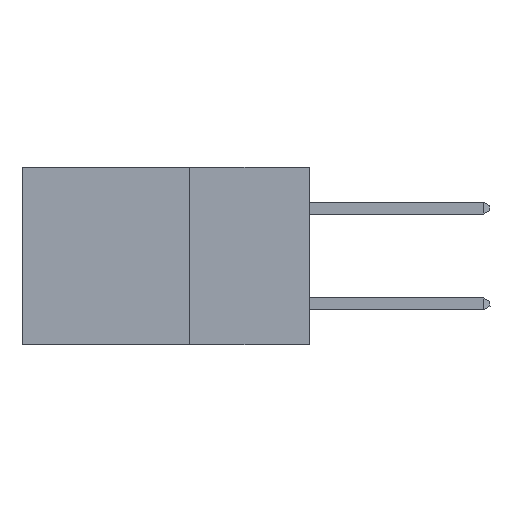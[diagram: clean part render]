
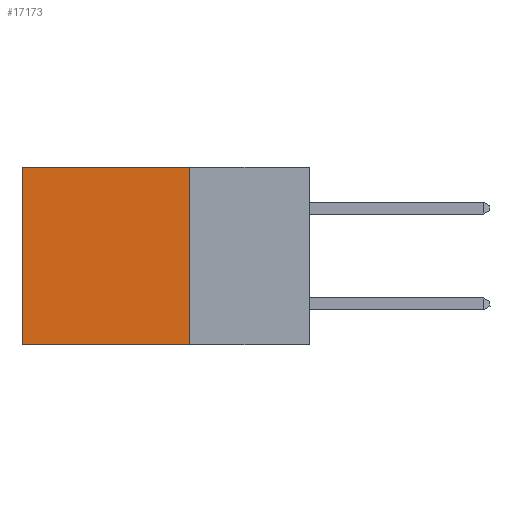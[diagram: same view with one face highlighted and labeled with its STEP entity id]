
A CAD part, left-side view. The second image highlights one B-rep face of the part: STEP entity #17173.
In plain terms, the highlighted planar face has unit normal (-1, 0, 0).
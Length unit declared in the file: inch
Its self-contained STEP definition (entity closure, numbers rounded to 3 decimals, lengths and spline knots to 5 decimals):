
#401 = CARTESIAN_POINT ( 'NONE',  ( 0.2875, 0.25, -0.37 ) ) ;
#508 = EDGE_CURVE ( 'NONE', #2702, #4521, #17261, .T. ) ;
#776 = VERTEX_POINT ( 'NONE', #10288 ) ;
#947 = EDGE_LOOP ( 'NONE', ( #15053, #12125, #2022, #2474 ) ) ;
#1586 = LINE ( 'NONE', #5569, #11376 ) ;
#1775 = PLANE ( 'NONE',  #7979 ) ;
#2022 = ORIENTED_EDGE ( 'NONE', *, *, #17127, .F. ) ;
#2103 = DIRECTION ( 'NONE',  ( 0., 0., -1. ) ) ;
#2354 = LINE ( 'NONE', #9148, #16115 ) ;
#2474 = ORIENTED_EDGE ( 'NONE', *, *, #10683, .T. ) ;
#2702 = VERTEX_POINT ( 'NONE', #15916 ) ;
#4402 = VECTOR ( 'NONE', #11416, 39.37008 ) ;
#4521 = VERTEX_POINT ( 'NONE', #14332 ) ;
#4786 = DIRECTION ( 'NONE',  ( 0., 0., -1. ) ) ;
#5569 = CARTESIAN_POINT ( 'NONE',  ( 0.2875, 0.25, 0. ) ) ;
#5970 = DIRECTION ( 'NONE',  ( 0., 1., 0. ) ) ;
#6257 = VERTEX_POINT ( 'NONE', #12027 ) ;
#7979 = AXIS2_PLACEMENT_3D ( 'NONE', #8861, #12738, #4786 ) ;
#8861 = CARTESIAN_POINT ( 'NONE',  ( 0.2875, 0.25, 0. ) ) ;
#9148 = CARTESIAN_POINT ( 'NONE',  ( 0.2875, 0.6, 0. ) ) ;
#9628 = DIRECTION ( 'NONE',  ( 0., 1., 0. ) ) ;
#10288 = CARTESIAN_POINT ( 'NONE',  ( 0.2875, 0.25, 0. ) ) ;
#10627 = VECTOR ( 'NONE', #5970, 39.37008 ) ;
#10683 = EDGE_CURVE ( 'NONE', #776, #6257, #1586, .T. ) ;
#11376 = VECTOR ( 'NONE', #9628, 39.37008 ) ;
#11416 = DIRECTION ( 'NONE',  ( 0., 0., -1. ) ) ;
#12027 = CARTESIAN_POINT ( 'NONE',  ( 0.2875, 0.6, 0. ) ) ;
#12125 = ORIENTED_EDGE ( 'NONE', *, *, #508, .F. ) ;
#12738 = DIRECTION ( 'NONE',  ( 1., 0., 0. ) ) ;
#14149 = FACE_OUTER_BOUND ( 'NONE', #947, .T. ) ;
#14332 = CARTESIAN_POINT ( 'NONE',  ( 0.2875, 0.6, -0.37 ) ) ;
#15053 = ORIENTED_EDGE ( 'NONE', *, *, #15868, .T. ) ;
#15134 = CARTESIAN_POINT ( 'NONE',  ( 0.2875, 0.25, 0. ) ) ;
#15868 = EDGE_CURVE ( 'NONE', #6257, #4521, #2354, .T. ) ;
#15916 = CARTESIAN_POINT ( 'NONE',  ( 0.2875, 0.25, -0.37 ) ) ;
#16115 = VECTOR ( 'NONE', #2103, 39.37008 ) ;
#16450 = LINE ( 'NONE', #15134, #4402 ) ;
#17127 = EDGE_CURVE ( 'NONE', #776, #2702, #16450, .T. ) ;
#17173 = ADVANCED_FACE ( 'NONE', ( #14149 ), #1775, .F. ) ;
#17261 = LINE ( 'NONE', #401, #10627 ) ;
